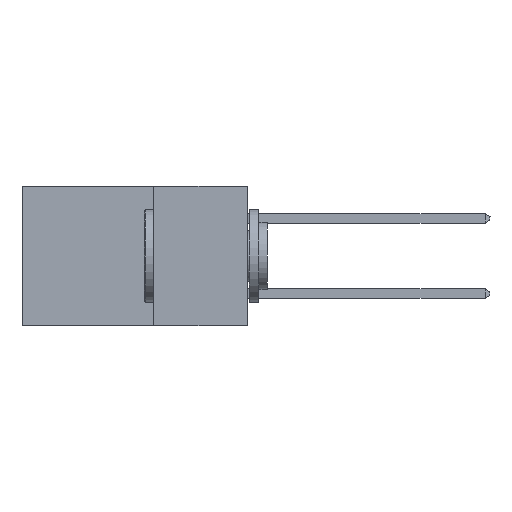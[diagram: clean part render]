
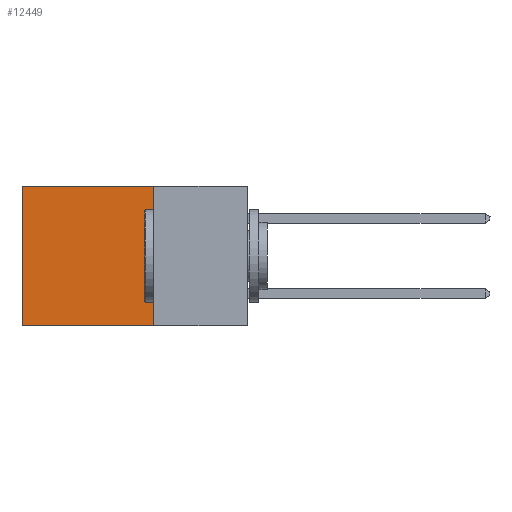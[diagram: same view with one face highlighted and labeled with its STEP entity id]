
A CAD part, left-side view. The second image highlights one B-rep face of the part: STEP entity #12449.
In plain terms, the highlighted planar face has unit normal (-1, 0, 0).
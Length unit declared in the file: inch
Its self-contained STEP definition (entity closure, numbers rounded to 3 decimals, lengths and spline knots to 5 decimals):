
#152 = CARTESIAN_POINT ( 'NONE',  ( 0.298, 0.6, -0.37 ) ) ;
#958 = ORIENTED_EDGE ( 'NONE', *, *, #7501, .F. ) ;
#1828 = PLANE ( 'NONE',  #16416 ) ;
#1943 = DIRECTION ( 'NONE',  ( 1., 0., 0. ) ) ;
#4265 = VERTEX_POINT ( 'NONE', #30071 ) ;
#6274 = CARTESIAN_POINT ( 'NONE',  ( 0.298, 0.25, 0. ) ) ;
#6286 = CARTESIAN_POINT ( 'NONE',  ( 0.298, 0.6, 0. ) ) ;
#6724 = LINE ( 'NONE', #6274, #26082 ) ;
#7119 = EDGE_CURVE ( 'NONE', #14700, #30815, #26971, .T. ) ;
#7501 = EDGE_CURVE ( 'NONE', #13383, #30815, #21898, .T. ) ;
#8588 = CARTESIAN_POINT ( 'NONE',  ( 0.298, 0.6, 0. ) ) ;
#8750 = DIRECTION ( 'NONE',  ( 0., 0., -1. ) ) ;
#8947 = CARTESIAN_POINT ( 'NONE',  ( 0.298, 0.25, -0.37 ) ) ;
#8978 = CARTESIAN_POINT ( 'NONE',  ( 0.298, 0.25, 0. ) ) ;
#10955 = EDGE_LOOP ( 'NONE', ( #31080, #958, #17534, #20096 ) ) ;
#12449 = ADVANCED_FACE ( 'NONE', ( #15339 ), #1828, .F. ) ;
#13191 = LINE ( 'NONE', #8978, #18401 ) ;
#13383 = VERTEX_POINT ( 'NONE', #8947 ) ;
#14700 = VERTEX_POINT ( 'NONE', #6286 ) ;
#14758 = EDGE_CURVE ( 'NONE', #4265, #14700, #13191, .T. ) ;
#15339 = FACE_OUTER_BOUND ( 'NONE', #10955, .T. ) ;
#16416 = AXIS2_PLACEMENT_3D ( 'NONE', #27077, #1943, #19676 ) ;
#16668 = DIRECTION ( 'NONE',  ( 0., 1., 0. ) ) ;
#17534 = ORIENTED_EDGE ( 'NONE', *, *, #29688, .F. ) ;
#18401 = VECTOR ( 'NONE', #16668, 39.37008 ) ;
#19676 = DIRECTION ( 'NONE',  ( 0., 0., -1. ) ) ;
#20096 = ORIENTED_EDGE ( 'NONE', *, *, #14758, .T. ) ;
#20165 = CARTESIAN_POINT ( 'NONE',  ( 0.298, 0.25, -0.37 ) ) ;
#21115 = VECTOR ( 'NONE', #32597, 39.37008 ) ;
#21143 = VECTOR ( 'NONE', #26304, 39.37008 ) ;
#21898 = LINE ( 'NONE', #20165, #21115 ) ;
#26082 = VECTOR ( 'NONE', #8750, 39.37008 ) ;
#26304 = DIRECTION ( 'NONE',  ( 0., 0., -1. ) ) ;
#26971 = LINE ( 'NONE', #8588, #21143 ) ;
#27077 = CARTESIAN_POINT ( 'NONE',  ( 0.298, 0.25, 0. ) ) ;
#29688 = EDGE_CURVE ( 'NONE', #4265, #13383, #6724, .T. ) ;
#30071 = CARTESIAN_POINT ( 'NONE',  ( 0.298, 0.25, 0. ) ) ;
#30815 = VERTEX_POINT ( 'NONE', #152 ) ;
#31080 = ORIENTED_EDGE ( 'NONE', *, *, #7119, .T. ) ;
#32597 = DIRECTION ( 'NONE',  ( 0., 1., 0. ) ) ;
